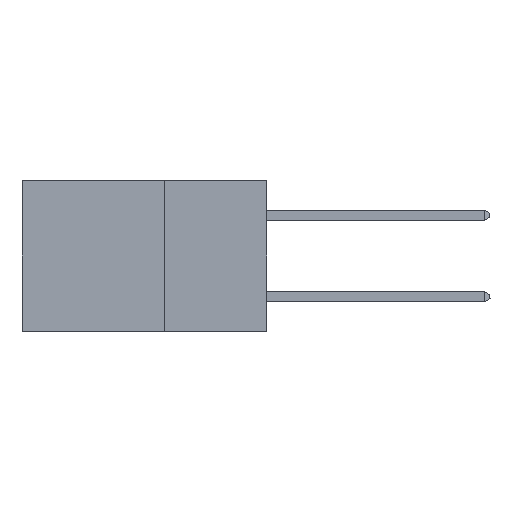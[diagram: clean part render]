
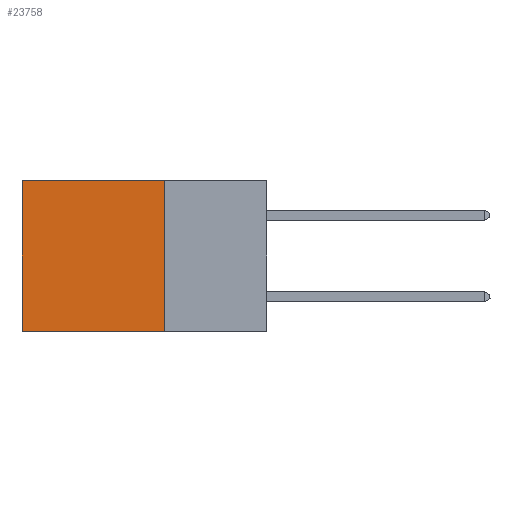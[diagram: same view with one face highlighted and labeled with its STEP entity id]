
A CAD part, left-side view. The second image highlights one B-rep face of the part: STEP entity #23758.
In plain terms, the highlighted planar face has unit normal (-1, 0, 0).
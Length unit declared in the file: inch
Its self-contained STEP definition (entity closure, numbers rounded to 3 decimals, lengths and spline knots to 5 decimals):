
#637 = EDGE_CURVE ( 'NONE', #6325, #7775, #7827, .T. ) ;
#1607 = EDGE_LOOP ( 'NONE', ( #23858, #35148, #41365, #35383 ) ) ;
#4797 = VERTEX_POINT ( 'NONE', #36585 ) ;
#5528 = VECTOR ( 'NONE', #15911, 39.37008 ) ;
#6274 = CARTESIAN_POINT ( 'NONE',  ( 0.2875, 0.25, 0. ) ) ;
#6325 = VERTEX_POINT ( 'NONE', #40608 ) ;
#7070 = LINE ( 'NONE', #6274, #5528 ) ;
#7351 = CARTESIAN_POINT ( 'NONE',  ( 0.2875, 0.6, 0. ) ) ;
#7775 = VERTEX_POINT ( 'NONE', #41778 ) ;
#7827 = LINE ( 'NONE', #11116, #20190 ) ;
#8634 = FACE_OUTER_BOUND ( 'NONE', #1607, .T. ) ;
#8950 = EDGE_CURVE ( 'NONE', #6325, #24862, #7070, .T. ) ;
#10658 = DIRECTION ( 'NONE',  ( 0., 0., -1. ) ) ;
#11116 = CARTESIAN_POINT ( 'NONE',  ( 0.2875, 0.25, 0. ) ) ;
#11643 = VECTOR ( 'NONE', #37576, 39.37008 ) ;
#13722 = PLANE ( 'NONE',  #39392 ) ;
#15911 = DIRECTION ( 'NONE',  ( 0., 0., -1. ) ) ;
#16763 = DIRECTION ( 'NONE',  ( 1., 0., 0. ) ) ;
#17915 = DIRECTION ( 'NONE',  ( 0., 1., 0. ) ) ;
#20190 = VECTOR ( 'NONE', #17915, 39.37008 ) ;
#22274 = CARTESIAN_POINT ( 'NONE',  ( 0.2875, 0.25, -0.37 ) ) ;
#22825 = LINE ( 'NONE', #7351, #42467 ) ;
#23235 = DIRECTION ( 'NONE',  ( 0., 0., -1. ) ) ;
#23758 = ADVANCED_FACE ( 'NONE', ( #8634 ), #13722, .F. ) ;
#23858 = ORIENTED_EDGE ( 'NONE', *, *, #29931, .T. ) ;
#24862 = VERTEX_POINT ( 'NONE', #22274 ) ;
#25365 = EDGE_CURVE ( 'NONE', #24862, #4797, #30245, .T. ) ;
#29931 = EDGE_CURVE ( 'NONE', #7775, #4797, #22825, .T. ) ;
#30245 = LINE ( 'NONE', #40573, #11643 ) ;
#35148 = ORIENTED_EDGE ( 'NONE', *, *, #25365, .F. ) ;
#35383 = ORIENTED_EDGE ( 'NONE', *, *, #637, .T. ) ;
#36557 = CARTESIAN_POINT ( 'NONE',  ( 0.2875, 0.25, 0. ) ) ;
#36585 = CARTESIAN_POINT ( 'NONE',  ( 0.2875, 0.6, -0.37 ) ) ;
#37576 = DIRECTION ( 'NONE',  ( 0., 1., 0. ) ) ;
#39392 = AXIS2_PLACEMENT_3D ( 'NONE', #36557, #16763, #23235 ) ;
#40573 = CARTESIAN_POINT ( 'NONE',  ( 0.2875, 0.25, -0.37 ) ) ;
#40608 = CARTESIAN_POINT ( 'NONE',  ( 0.2875, 0.25, 0. ) ) ;
#41365 = ORIENTED_EDGE ( 'NONE', *, *, #8950, .F. ) ;
#41778 = CARTESIAN_POINT ( 'NONE',  ( 0.2875, 0.6, 0. ) ) ;
#42467 = VECTOR ( 'NONE', #10658, 39.37008 ) ;
